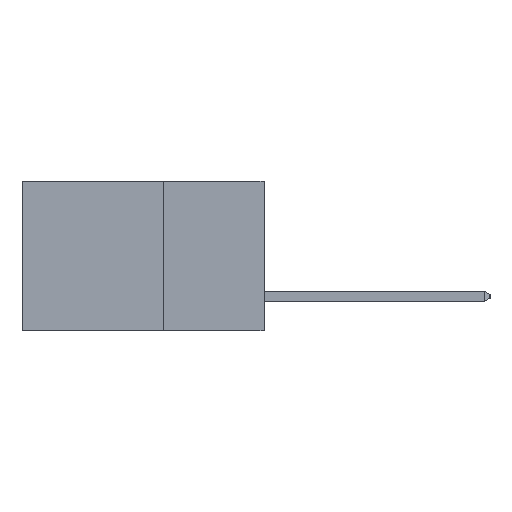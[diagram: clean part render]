
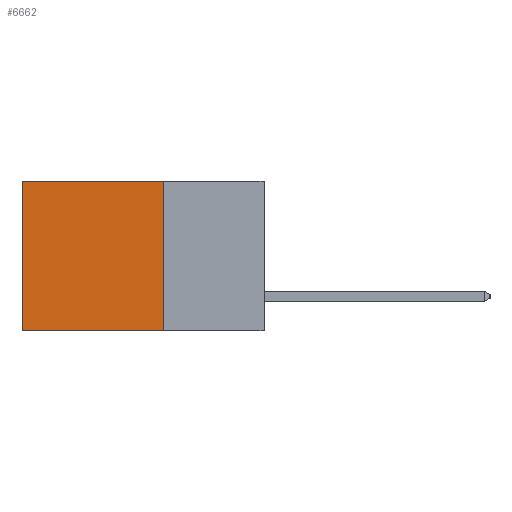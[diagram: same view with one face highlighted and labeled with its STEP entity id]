
A CAD part, left-side view. The second image highlights one B-rep face of the part: STEP entity #6662.
In plain terms, the highlighted planar face has unit normal (-1, 0, 0).
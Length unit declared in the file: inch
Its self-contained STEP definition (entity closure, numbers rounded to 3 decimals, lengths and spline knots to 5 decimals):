
#159 = VECTOR ( 'NONE', #5381, 39.37008 ) ;
#264 = LINE ( 'NONE', #5951, #13287 ) ;
#2417 = CARTESIAN_POINT ( 'NONE',  ( 0.2615, 0.25, -0.37 ) ) ;
#3060 = VERTEX_POINT ( 'NONE', #8607 ) ;
#3477 = EDGE_LOOP ( 'NONE', ( #14627, #12428, #11709, #7026 ) ) ;
#3551 = VERTEX_POINT ( 'NONE', #13656 ) ;
#4978 = VECTOR ( 'NONE', #16408, 39.37008 ) ;
#4997 = EDGE_CURVE ( 'NONE', #3551, #3060, #11782, .T. ) ;
#5381 = DIRECTION ( 'NONE',  ( 0., 0., -1. ) ) ;
#5951 = CARTESIAN_POINT ( 'NONE',  ( 0.2615, 0.25, 0. ) ) ;
#6333 = DIRECTION ( 'NONE',  ( 1., 0., 0. ) ) ;
#6662 = ADVANCED_FACE ( 'NONE', ( #10740 ), #13885, .F. ) ;
#7026 = ORIENTED_EDGE ( 'NONE', *, *, #9903, .T. ) ;
#8607 = CARTESIAN_POINT ( 'NONE',  ( 0.2615, 0.25, -0.37 ) ) ;
#8867 = DIRECTION ( 'NONE',  ( 0., 1., 0. ) ) ;
#8875 = CARTESIAN_POINT ( 'NONE',  ( 0.2615, 0.25, -0.37 ) ) ;
#9887 = LINE ( 'NONE', #16186, #10670 ) ;
#9895 = CARTESIAN_POINT ( 'NONE',  ( 0.2615, 0.6, 0. ) ) ;
#9903 = EDGE_CURVE ( 'NONE', #3551, #12860, #264, .T. ) ;
#10670 = VECTOR ( 'NONE', #8867, 39.37008 ) ;
#10740 = FACE_OUTER_BOUND ( 'NONE', #3477, .T. ) ;
#10999 = DIRECTION ( 'NONE',  ( 0., 1., 0. ) ) ;
#11633 = EDGE_CURVE ( 'NONE', #3060, #15758, #9887, .T. ) ;
#11709 = ORIENTED_EDGE ( 'NONE', *, *, #4997, .F. ) ;
#11782 = LINE ( 'NONE', #2417, #4978 ) ;
#12428 = ORIENTED_EDGE ( 'NONE', *, *, #11633, .F. ) ;
#12468 = EDGE_CURVE ( 'NONE', #12860, #15758, #16344, .T. ) ;
#12860 = VERTEX_POINT ( 'NONE', #9895 ) ;
#12893 = CARTESIAN_POINT ( 'NONE',  ( 0.2615, 0.6, -0.37 ) ) ;
#12978 = CARTESIAN_POINT ( 'NONE',  ( 0.2615, 0.6, -0.37 ) ) ;
#13287 = VECTOR ( 'NONE', #10999, 39.37008 ) ;
#13656 = CARTESIAN_POINT ( 'NONE',  ( 0.2615, 0.25, 0. ) ) ;
#13885 = PLANE ( 'NONE',  #16479 ) ;
#14627 = ORIENTED_EDGE ( 'NONE', *, *, #12468, .T. ) ;
#15082 = DIRECTION ( 'NONE',  ( 0., 0., -1. ) ) ;
#15758 = VERTEX_POINT ( 'NONE', #12893 ) ;
#16186 = CARTESIAN_POINT ( 'NONE',  ( 0.2615, 0.25, -0.37 ) ) ;
#16344 = LINE ( 'NONE', #12978, #159 ) ;
#16408 = DIRECTION ( 'NONE',  ( 0., 0., -1. ) ) ;
#16479 = AXIS2_PLACEMENT_3D ( 'NONE', #8875, #6333, #15082 ) ;
